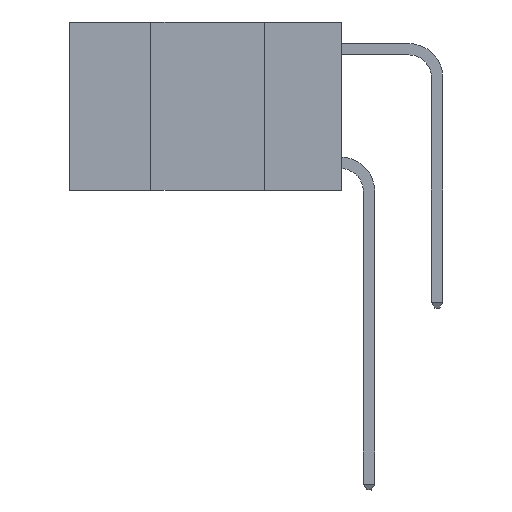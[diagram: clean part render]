
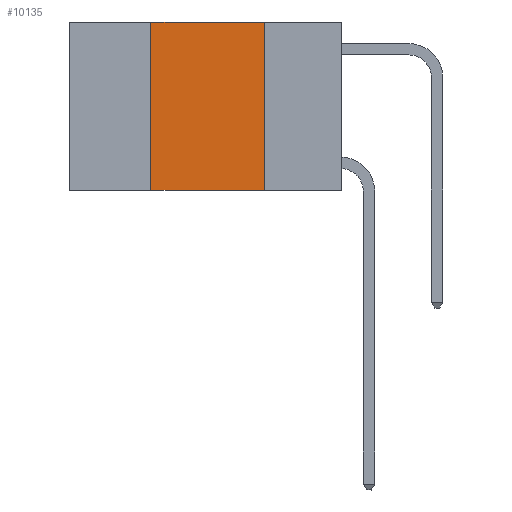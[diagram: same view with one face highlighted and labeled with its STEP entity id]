
A CAD part, left-side view. The second image highlights one B-rep face of the part: STEP entity #10135.
In plain terms, the highlighted planar face has unit normal (-1, 0, 0).
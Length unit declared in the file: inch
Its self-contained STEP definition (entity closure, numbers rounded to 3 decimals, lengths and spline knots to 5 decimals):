
#158 = LINE ( 'NONE', #12381, #2716 ) ;
#442 = DIRECTION ( 'NONE',  ( 0., 0., -1. ) ) ;
#498 = CARTESIAN_POINT ( 'NONE',  ( 0., 0.6, 0. ) ) ;
#1523 = AXIS2_PLACEMENT_3D ( 'NONE', #10717, #6705, #442 ) ;
#2327 = CARTESIAN_POINT ( 'NONE',  ( 0., 0.42, -0.37 ) ) ;
#2565 = PLANE ( 'NONE',  #1523 ) ;
#2716 = VECTOR ( 'NONE', #7392, 39.37008 ) ;
#2932 = CARTESIAN_POINT ( 'NONE',  ( 0., 0.42, 0. ) ) ;
#3977 = EDGE_CURVE ( 'NONE', #9016, #6279, #5849, .T. ) ;
#4440 = VERTEX_POINT ( 'NONE', #10503 ) ;
#4901 = VECTOR ( 'NONE', #10684, 39.37008 ) ;
#5847 = CARTESIAN_POINT ( 'NONE',  ( 0., 0.17, 0. ) ) ;
#5849 = LINE ( 'NONE', #9647, #4901 ) ;
#5936 = EDGE_CURVE ( 'NONE', #4440, #9016, #11175, .T. ) ;
#6279 = VERTEX_POINT ( 'NONE', #10317 ) ;
#6705 = DIRECTION ( 'NONE',  ( 1., 0., 0. ) ) ;
#7060 = DIRECTION ( 'NONE',  ( 0., 0., 1. ) ) ;
#7392 = DIRECTION ( 'NONE',  ( 0., -1., 0. ) ) ;
#7761 = DIRECTION ( 'NONE',  ( 0., -1., 0. ) ) ;
#7856 = VECTOR ( 'NONE', #7060, 39.37008 ) ;
#8252 = VERTEX_POINT ( 'NONE', #2327 ) ;
#8475 = VECTOR ( 'NONE', #7761, 39.37008 ) ;
#8598 = EDGE_LOOP ( 'NONE', ( #10968, #11967, #8892, #9590 ) ) ;
#8892 = ORIENTED_EDGE ( 'NONE', *, *, #11635, .F. ) ;
#9016 = VERTEX_POINT ( 'NONE', #5847 ) ;
#9590 = ORIENTED_EDGE ( 'NONE', *, *, #12969, .T. ) ;
#9647 = CARTESIAN_POINT ( 'NONE',  ( 0., 0.17, 0. ) ) ;
#9792 = FACE_OUTER_BOUND ( 'NONE', #8598, .T. ) ;
#10135 = ADVANCED_FACE ( 'NONE', ( #9792 ), #2565, .F. ) ;
#10317 = CARTESIAN_POINT ( 'NONE',  ( 0., 0.17, -0.37 ) ) ;
#10503 = CARTESIAN_POINT ( 'NONE',  ( 0., 0.42, 0. ) ) ;
#10561 = LINE ( 'NONE', #2932, #7856 ) ;
#10684 = DIRECTION ( 'NONE',  ( 0., 0., -1. ) ) ;
#10717 = CARTESIAN_POINT ( 'NONE',  ( 0., 0.6, 0. ) ) ;
#10968 = ORIENTED_EDGE ( 'NONE', *, *, #3977, .F. ) ;
#11175 = LINE ( 'NONE', #498, #8475 ) ;
#11635 = EDGE_CURVE ( 'NONE', #8252, #4440, #10561, .T. ) ;
#11967 = ORIENTED_EDGE ( 'NONE', *, *, #5936, .F. ) ;
#12381 = CARTESIAN_POINT ( 'NONE',  ( 0., 0.6, -0.37 ) ) ;
#12969 = EDGE_CURVE ( 'NONE', #8252, #6279, #158, .T. ) ;
